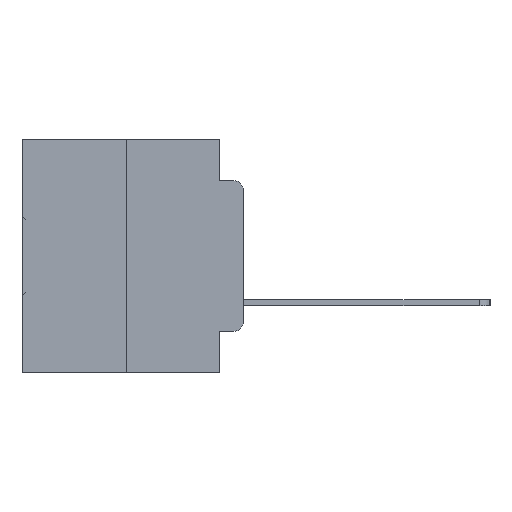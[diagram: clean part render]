
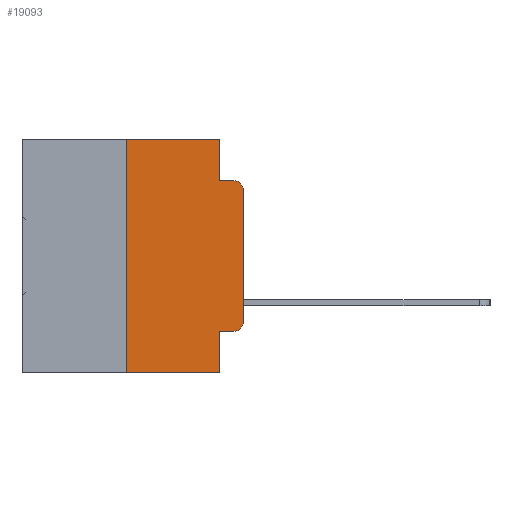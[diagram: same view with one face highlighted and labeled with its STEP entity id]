
A CAD part, left-side view. The second image highlights one B-rep face of the part: STEP entity #19093.
In plain terms, the highlighted planar face has unit normal (-1, 0, 0).
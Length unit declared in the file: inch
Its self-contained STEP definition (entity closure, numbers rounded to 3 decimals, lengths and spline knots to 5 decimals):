
#41 = VECTOR ( 'NONE', #20620, 39.37008 ) ;
#393 = VECTOR ( 'NONE', #4411, 39.37008 ) ;
#426 = VERTEX_POINT ( 'NONE', #7541 ) ;
#630 = CARTESIAN_POINT ( 'NONE',  ( 0., 0.051, -0.0885 ) ) ;
#763 = PLANE ( 'NONE',  #21201 ) ;
#823 = CARTESIAN_POINT ( 'NONE',  ( 0., 0.02, -0.1085 ) ) ;
#1056 = VERTEX_POINT ( 'NONE', #15916 ) ;
#1184 = VERTEX_POINT ( 'NONE', #32626 ) ;
#1747 = VERTEX_POINT ( 'NONE', #10309 ) ;
#1777 = EDGE_LOOP ( 'NONE', ( #30347, #31950, #32757, #27567, #21566, #22350, #10196, #23983, #11853, #18747 ) ) ;
#2596 = VECTOR ( 'NONE', #5885, 39.37008 ) ;
#3551 = DIRECTION ( 'NONE',  ( 0., 0., -1. ) ) ;
#3612 = EDGE_CURVE ( 'NONE', #14249, #16791, #32029, .T. ) ;
#4321 = VERTEX_POINT ( 'NONE', #33605 ) ;
#4411 = DIRECTION ( 'NONE',  ( 0., 0., 1. ) ) ;
#4662 = EDGE_CURVE ( 'NONE', #1056, #17193, #15525, .T. ) ;
#5660 = DIRECTION ( 'NONE',  ( -1., 0., 0. ) ) ;
#5885 = DIRECTION ( 'NONE',  ( 0., 0., -1. ) ) ;
#6258 = DIRECTION ( 'NONE',  ( 1., 0., 0. ) ) ;
#6615 = DIRECTION ( 'NONE',  ( 0., -1., 0. ) ) ;
#6799 = LINE ( 'NONE', #30566, #393 ) ;
#7541 = CARTESIAN_POINT ( 'NONE',  ( 0., 0.25, -0.5 ) ) ;
#9185 = VECTOR ( 'NONE', #18225, 39.37008 ) ;
#9382 = DIRECTION ( 'NONE',  ( 0., 0., 1. ) ) ;
#10196 = ORIENTED_EDGE ( 'NONE', *, *, #19143, .T. ) ;
#10309 = CARTESIAN_POINT ( 'NONE',  ( 0., 0.051, -0.5 ) ) ;
#11229 = EDGE_CURVE ( 'NONE', #426, #1184, #6799, .T. ) ;
#11373 = CARTESIAN_POINT ( 'NONE',  ( 0., 0.051, 0. ) ) ;
#11853 = ORIENTED_EDGE ( 'NONE', *, *, #3612, .T. ) ;
#12139 = EDGE_CURVE ( 'NONE', #16791, #4321, #26785, .T. ) ;
#12760 = LINE ( 'NONE', #18123, #41 ) ;
#13362 = VECTOR ( 'NONE', #27036, 39.37008 ) ;
#13725 = EDGE_CURVE ( 'NONE', #1184, #27929, #22216, .T. ) ;
#14174 = LINE ( 'NONE', #19269, #13362 ) ;
#14213 = CARTESIAN_POINT ( 'NONE',  ( 0., 0.473, 0. ) ) ;
#14249 = VERTEX_POINT ( 'NONE', #14454 ) ;
#14454 = CARTESIAN_POINT ( 'NONE',  ( 0., 0.051, -0.4115 ) ) ;
#14825 = VERTEX_POINT ( 'NONE', #630 ) ;
#15525 = CIRCLE ( 'NONE', #33260, 0.02 ) ;
#15916 = CARTESIAN_POINT ( 'NONE',  ( 0., 0., -0.1085 ) ) ;
#16791 = VERTEX_POINT ( 'NONE', #29746 ) ;
#17193 = VERTEX_POINT ( 'NONE', #31403 ) ;
#17615 = VECTOR ( 'NONE', #25279, 39.37008 ) ;
#17868 = VECTOR ( 'NONE', #6615, 39.37008 ) ;
#18123 = CARTESIAN_POINT ( 'NONE',  ( 0., 0.051, -0.0885 ) ) ;
#18225 = DIRECTION ( 'NONE',  ( 0., -1., 0. ) ) ;
#18747 = ORIENTED_EDGE ( 'NONE', *, *, #12139, .T. ) ;
#18792 = CARTESIAN_POINT ( 'NONE',  ( 0., 0.051, 0. ) ) ;
#19093 = ADVANCED_FACE ( 'NONE', ( #26320 ), #763, .F. ) ;
#19143 = EDGE_CURVE ( 'NONE', #426, #1747, #24699, .T. ) ;
#19269 = CARTESIAN_POINT ( 'NONE',  ( 0., 0.051, 0. ) ) ;
#19486 = DIRECTION ( 'NONE',  ( -1., 0., 0. ) ) ;
#20240 = CARTESIAN_POINT ( 'NONE',  ( 0., 0.051, -0.4115 ) ) ;
#20446 = LINE ( 'NONE', #30061, #33237 ) ;
#20620 = DIRECTION ( 'NONE',  ( 0., -1., 0. ) ) ;
#21201 = AXIS2_PLACEMENT_3D ( 'NONE', #14213, #6258, #24604 ) ;
#21464 = CARTESIAN_POINT ( 'NONE',  ( 0., 0.02, -0.3915 ) ) ;
#21566 = ORIENTED_EDGE ( 'NONE', *, *, #13725, .F. ) ;
#22216 = LINE ( 'NONE', #25982, #9185 ) ;
#22350 = ORIENTED_EDGE ( 'NONE', *, *, #11229, .F. ) ;
#23555 = AXIS2_PLACEMENT_3D ( 'NONE', #21464, #5660, #24051 ) ;
#23983 = ORIENTED_EDGE ( 'NONE', *, *, #28612, .F. ) ;
#24051 = DIRECTION ( 'NONE',  ( 0., 0., -1. ) ) ;
#24604 = DIRECTION ( 'NONE',  ( 0., 0., -1. ) ) ;
#24699 = LINE ( 'NONE', #29946, #17868 ) ;
#25279 = DIRECTION ( 'NONE',  ( 0., -1., 0. ) ) ;
#25982 = CARTESIAN_POINT ( 'NONE',  ( 0., 0.473, 0. ) ) ;
#26320 = FACE_OUTER_BOUND ( 'NONE', #1777, .T. ) ;
#26785 = CIRCLE ( 'NONE', #23555, 0.02 ) ;
#27036 = DIRECTION ( 'NONE',  ( 0., 0., -1. ) ) ;
#27567 = ORIENTED_EDGE ( 'NONE', *, *, #29099, .F. ) ;
#27929 = VERTEX_POINT ( 'NONE', #18792 ) ;
#28612 = EDGE_CURVE ( 'NONE', #14249, #1747, #30487, .T. ) ;
#29099 = EDGE_CURVE ( 'NONE', #27929, #14825, #14174, .T. ) ;
#29746 = CARTESIAN_POINT ( 'NONE',  ( 0., 0.02, -0.4115 ) ) ;
#29946 = CARTESIAN_POINT ( 'NONE',  ( 0., 0.473, -0.5 ) ) ;
#30061 = CARTESIAN_POINT ( 'NONE',  ( 0., 0., 0. ) ) ;
#30347 = ORIENTED_EDGE ( 'NONE', *, *, #33028, .T. ) ;
#30487 = LINE ( 'NONE', #11373, #2596 ) ;
#30566 = CARTESIAN_POINT ( 'NONE',  ( 0., 0.25, 0. ) ) ;
#31403 = CARTESIAN_POINT ( 'NONE',  ( 0., 0.02, -0.0885 ) ) ;
#31950 = ORIENTED_EDGE ( 'NONE', *, *, #4662, .T. ) ;
#32029 = LINE ( 'NONE', #20240, #17615 ) ;
#32626 = CARTESIAN_POINT ( 'NONE',  ( 0., 0.25, 0. ) ) ;
#32635 = EDGE_CURVE ( 'NONE', #14825, #17193, #12760, .T. ) ;
#32757 = ORIENTED_EDGE ( 'NONE', *, *, #32635, .F. ) ;
#33028 = EDGE_CURVE ( 'NONE', #4321, #1056, #20446, .T. ) ;
#33237 = VECTOR ( 'NONE', #9382, 39.37008 ) ;
#33260 = AXIS2_PLACEMENT_3D ( 'NONE', #823, #19486, #3551 ) ;
#33605 = CARTESIAN_POINT ( 'NONE',  ( 0., 0., -0.3915 ) ) ;
